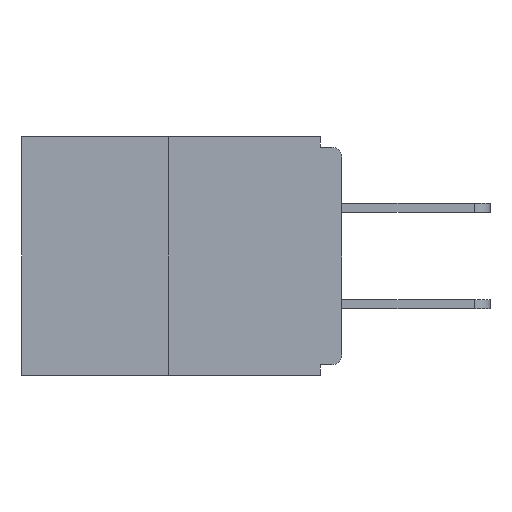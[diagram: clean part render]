
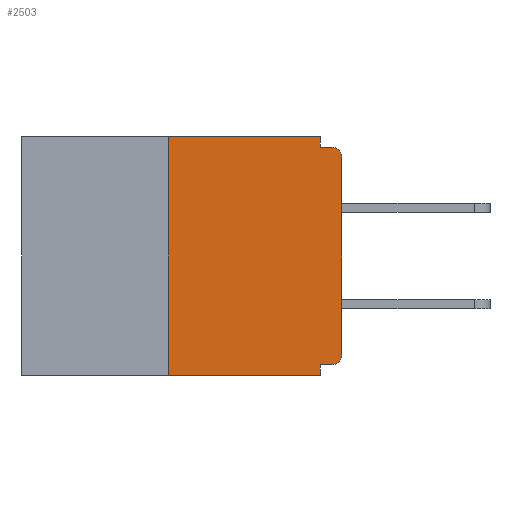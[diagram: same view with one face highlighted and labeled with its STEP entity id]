
A CAD part, left-side view. The second image highlights one B-rep face of the part: STEP entity #2503.
In plain terms, the highlighted planar face has unit normal (-1, 0, 0).
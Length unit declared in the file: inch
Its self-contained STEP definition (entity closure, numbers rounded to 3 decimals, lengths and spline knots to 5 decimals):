
#427 = CIRCLE ( 'NONE', #3210, 0.015 ) ;
#458 = AXIS2_PLACEMENT_3D ( 'NONE', #18179, #13314, #6528 ) ;
#710 = DIRECTION ( 'NONE',  ( 0., 0., -1. ) ) ;
#780 = EDGE_CURVE ( 'NONE', #11660, #16479, #427, .T. ) ;
#808 = EDGE_CURVE ( 'NONE', #19324, #16825, #5902, .T. ) ;
#1005 = VECTOR ( 'NONE', #20360, 39.37008 ) ;
#1183 = VECTOR ( 'NONE', #14005, 39.37008 ) ;
#1275 = LINE ( 'NONE', #18167, #17740 ) ;
#1506 = CARTESIAN_POINT ( 'NONE',  ( 0., 0., -0.015 ) ) ;
#1718 = ORIENTED_EDGE ( 'NONE', *, *, #19567, .F. ) ;
#1999 = CARTESIAN_POINT ( 'NONE',  ( 0., 0., -0.313 ) ) ;
#2391 = DIRECTION ( 'NONE',  ( 0., 0., -1. ) ) ;
#2503 = ADVANCED_FACE ( 'NONE', ( #4587 ), #7101, .F. ) ;
#2547 = CARTESIAN_POINT ( 'NONE',  ( 0., 0.46, 0. ) ) ;
#2559 = CARTESIAN_POINT ( 'NONE',  ( 0., 0., -0.328 ) ) ;
#3180 = EDGE_CURVE ( 'NONE', #16479, #7504, #11404, .T. ) ;
#3210 = AXIS2_PLACEMENT_3D ( 'NONE', #12904, #21645, #2391 ) ;
#3587 = CARTESIAN_POINT ( 'NONE',  ( 0., 0.015, -0.328 ) ) ;
#4085 = VERTEX_POINT ( 'NONE', #9178 ) ;
#4357 = DIRECTION ( 'NONE',  ( 0., -1., 0. ) ) ;
#4587 = FACE_OUTER_BOUND ( 'NONE', #17884, .T. ) ;
#4619 = CARTESIAN_POINT ( 'NONE',  ( 0., 0., 0. ) ) ;
#4657 = CARTESIAN_POINT ( 'NONE',  ( 0., 0.25, 0. ) ) ;
#4854 = ORIENTED_EDGE ( 'NONE', *, *, #18170, .T. ) ;
#4984 = LINE ( 'NONE', #5177, #14879 ) ;
#5177 = CARTESIAN_POINT ( 'NONE',  ( 0., 0.25, 0. ) ) ;
#5263 = VECTOR ( 'NONE', #20237, 39.37008 ) ;
#5299 = LINE ( 'NONE', #1506, #1183 ) ;
#5902 = LINE ( 'NONE', #2547, #12763 ) ;
#6528 = DIRECTION ( 'NONE',  ( 0., 0., -1. ) ) ;
#6734 = CARTESIAN_POINT ( 'NONE',  ( 0., 0.031, -0.328 ) ) ;
#7101 = PLANE ( 'NONE',  #458 ) ;
#7226 = CARTESIAN_POINT ( 'NONE',  ( 0., 0.25, -0.343 ) ) ;
#7504 = VERTEX_POINT ( 'NONE', #10591 ) ;
#7782 = DIRECTION ( 'NONE',  ( 0., 0., -1. ) ) ;
#7922 = ORIENTED_EDGE ( 'NONE', *, *, #808, .F. ) ;
#8014 = CARTESIAN_POINT ( 'NONE',  ( 0., 0.031, 0. ) ) ;
#8264 = LINE ( 'NONE', #2559, #18704 ) ;
#8734 = EDGE_CURVE ( 'NONE', #16441, #19324, #4984, .T. ) ;
#9063 = EDGE_CURVE ( 'NONE', #16441, #4085, #22266, .T. ) ;
#9178 = CARTESIAN_POINT ( 'NONE',  ( 0., 0.031, -0.343 ) ) ;
#9180 = EDGE_CURVE ( 'NONE', #11660, #11575, #8264, .T. ) ;
#9993 = ORIENTED_EDGE ( 'NONE', *, *, #780, .T. ) ;
#10089 = VERTEX_POINT ( 'NONE', #19185 ) ;
#10591 = CARTESIAN_POINT ( 'NONE',  ( 0., 0., -0.03 ) ) ;
#10726 = ORIENTED_EDGE ( 'NONE', *, *, #15216, .F. ) ;
#11023 = ORIENTED_EDGE ( 'NONE', *, *, #15116, .F. ) ;
#11171 = DIRECTION ( 'NONE',  ( -1., 0., 0. ) ) ;
#11277 = DIRECTION ( 'NONE',  ( 0., 1., 0. ) ) ;
#11404 = LINE ( 'NONE', #4619, #1005 ) ;
#11575 = VERTEX_POINT ( 'NONE', #6734 ) ;
#11660 = VERTEX_POINT ( 'NONE', #3587 ) ;
#12197 = CARTESIAN_POINT ( 'NONE',  ( 0., 0.031, -0.015 ) ) ;
#12763 = VECTOR ( 'NONE', #4357, 39.37008 ) ;
#12904 = CARTESIAN_POINT ( 'NONE',  ( 0., 0.015, -0.313 ) ) ;
#13040 = CARTESIAN_POINT ( 'NONE',  ( 0., 0.46, -0.343 ) ) ;
#13314 = DIRECTION ( 'NONE',  ( 1., 0., 0. ) ) ;
#13520 = ORIENTED_EDGE ( 'NONE', *, *, #9180, .F. ) ;
#14005 = DIRECTION ( 'NONE',  ( 0., -1., 0. ) ) ;
#14159 = DIRECTION ( 'NONE',  ( 0., 0., -1. ) ) ;
#14519 = ORIENTED_EDGE ( 'NONE', *, *, #9063, .T. ) ;
#14879 = VECTOR ( 'NONE', #18713, 39.37008 ) ;
#15116 = EDGE_CURVE ( 'NONE', #16301, #10089, #5299, .T. ) ;
#15216 = EDGE_CURVE ( 'NONE', #16825, #16301, #22042, .T. ) ;
#15286 = ORIENTED_EDGE ( 'NONE', *, *, #3180, .T. ) ;
#16291 = VECTOR ( 'NONE', #14159, 39.37008 ) ;
#16301 = VERTEX_POINT ( 'NONE', #12197 ) ;
#16441 = VERTEX_POINT ( 'NONE', #7226 ) ;
#16479 = VERTEX_POINT ( 'NONE', #1999 ) ;
#16766 = ORIENTED_EDGE ( 'NONE', *, *, #8734, .F. ) ;
#16825 = VERTEX_POINT ( 'NONE', #8014 ) ;
#17700 = CARTESIAN_POINT ( 'NONE',  ( 0., 0.031, 0. ) ) ;
#17740 = VECTOR ( 'NONE', #7782, 39.37008 ) ;
#17884 = EDGE_LOOP ( 'NONE', ( #7922, #16766, #14519, #1718, #13520, #9993, #15286, #4854, #11023, #10726 ) ) ;
#18167 = CARTESIAN_POINT ( 'NONE',  ( 0., 0.031, -0.343 ) ) ;
#18170 = EDGE_CURVE ( 'NONE', #7504, #10089, #18350, .T. ) ;
#18179 = CARTESIAN_POINT ( 'NONE',  ( 0., 0.46, 0. ) ) ;
#18350 = CIRCLE ( 'NONE', #20350, 0.015 ) ;
#18704 = VECTOR ( 'NONE', #11277, 39.37008 ) ;
#18713 = DIRECTION ( 'NONE',  ( 0., 0., 1. ) ) ;
#19185 = CARTESIAN_POINT ( 'NONE',  ( 0., 0.015, -0.015 ) ) ;
#19324 = VERTEX_POINT ( 'NONE', #4657 ) ;
#19567 = EDGE_CURVE ( 'NONE', #11575, #4085, #1275, .T. ) ;
#19939 = CARTESIAN_POINT ( 'NONE',  ( 0., 0.015, -0.03 ) ) ;
#20237 = DIRECTION ( 'NONE',  ( 0., -1., 0. ) ) ;
#20350 = AXIS2_PLACEMENT_3D ( 'NONE', #19939, #11171, #710 ) ;
#20360 = DIRECTION ( 'NONE',  ( 0., 0., 1. ) ) ;
#21645 = DIRECTION ( 'NONE',  ( -1., 0., 0. ) ) ;
#22042 = LINE ( 'NONE', #17700, #16291 ) ;
#22266 = LINE ( 'NONE', #13040, #5263 ) ;
